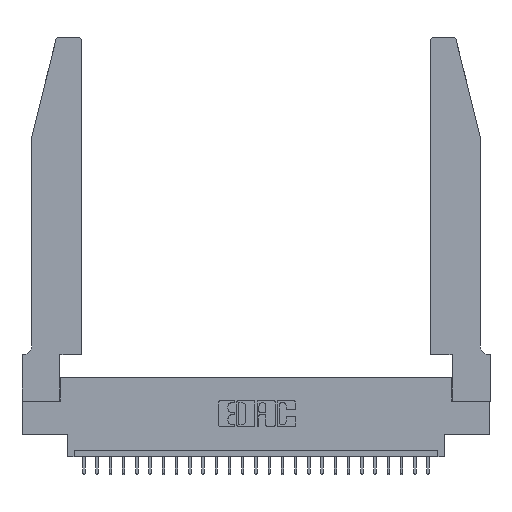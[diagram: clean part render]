
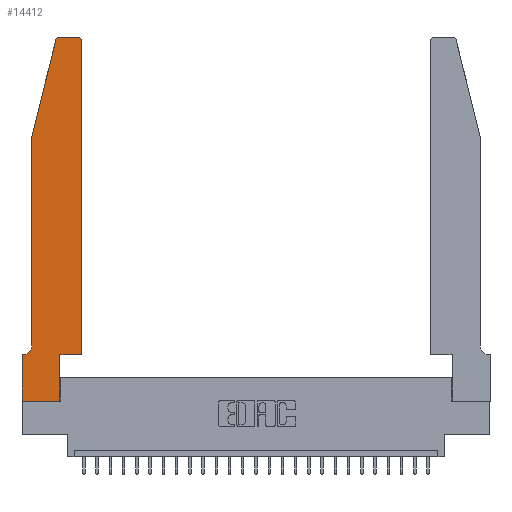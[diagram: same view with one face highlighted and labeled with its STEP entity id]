
A CAD part, top view. The second image highlights one B-rep face of the part: STEP entity #14412.
In plain terms, the highlighted planar face has unit normal (0, 0, 1).
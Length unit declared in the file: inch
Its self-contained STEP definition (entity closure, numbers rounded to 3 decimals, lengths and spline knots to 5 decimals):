
#341 = DIRECTION ( 'NONE',  ( 0., -1., 0. ) ) ;
#376 = ORIENTED_EDGE ( 'NONE', *, *, #8620, .T. ) ;
#528 = AXIS2_PLACEMENT_3D ( 'NONE', #14301, #6112, #1707 ) ;
#694 = EDGE_CURVE ( 'NONE', #7402, #24415, #25344, .T. ) ;
#787 = DIRECTION ( 'NONE',  ( -1., 0., 0. ) ) ;
#813 = CIRCLE ( 'NONE', #26878, 0.03 ) ;
#1213 = ORIENTED_EDGE ( 'NONE', *, *, #19208, .T. ) ;
#1426 = ORIENTED_EDGE ( 'NONE', *, *, #20677, .T. ) ;
#1485 = DIRECTION ( 'NONE',  ( 0., 1., 0. ) ) ;
#1707 = DIRECTION ( 'NONE',  ( 1., 0., 0. ) ) ;
#2209 = VERTEX_POINT ( 'NONE', #5095 ) ;
#2527 = CARTESIAN_POINT ( 'NONE',  ( 0.0755, 2., 0.37 ) ) ;
#3108 = VECTOR ( 'NONE', #8876, 39.37008 ) ;
#3125 = VECTOR ( 'NONE', #4158, 39.37008 ) ;
#3211 = EDGE_CURVE ( 'NONE', #4930, #22419, #3374, .T. ) ;
#3374 = LINE ( 'NONE', #16077, #22943 ) ;
#3645 = CARTESIAN_POINT ( 'NONE',  ( 0.2865, 0.35, 0.37 ) ) ;
#3702 = DIRECTION ( 'NONE',  ( -1., 0., 0. ) ) ;
#3962 = AXIS2_PLACEMENT_3D ( 'NONE', #18215, #22082, #3702 ) ;
#4158 = DIRECTION ( 'NONE',  ( -1., 0., 0. ) ) ;
#4218 = LINE ( 'NONE', #25383, #10726 ) ;
#4930 = VERTEX_POINT ( 'NONE', #3645 ) ;
#5095 = CARTESIAN_POINT ( 'NONE',  ( 0., 0., 0.37 ) ) ;
#5184 = EDGE_LOOP ( 'NONE', ( #8796, #376, #10819, #16436, #1213, #1426, #23191, #9444, #22087, #20140, #8868, #13219 ) ) ;
#5311 = CARTESIAN_POINT ( 'NONE',  ( 0.0755, 0.42, 0.37 ) ) ;
#5367 = LINE ( 'NONE', #26244, #21710 ) ;
#5910 = CARTESIAN_POINT ( 'NONE',  ( 0.4505, 0.35, 0.37 ) ) ;
#5990 = FACE_OUTER_BOUND ( 'NONE', #5184, .T. ) ;
#6112 = DIRECTION ( 'NONE',  ( 0., 0., 1. ) ) ;
#6218 = AXIS2_PLACEMENT_3D ( 'NONE', #20593, #25018, #20462 ) ;
#7402 = VERTEX_POINT ( 'NONE', #24793 ) ;
#7580 = VECTOR ( 'NONE', #14351, 39.37008 ) ;
#7696 = LINE ( 'NONE', #26513, #27016 ) ;
#8125 = VERTEX_POINT ( 'NONE', #22110 ) ;
#8146 = VERTEX_POINT ( 'NONE', #24330 ) ;
#8329 = DIRECTION ( 'NONE',  ( 1., 0., 0. ) ) ;
#8620 = EDGE_CURVE ( 'NONE', #8125, #7402, #813, .T. ) ;
#8796 = ORIENTED_EDGE ( 'NONE', *, *, #23395, .T. ) ;
#8868 = ORIENTED_EDGE ( 'NONE', *, *, #8987, .T. ) ;
#8876 = DIRECTION ( 'NONE',  ( -0.239, -0.971, 0. ) ) ;
#8987 = EDGE_CURVE ( 'NONE', #22419, #26994, #13859, .T. ) ;
#9112 = CARTESIAN_POINT ( 'NONE',  ( 0., 0.35, 0.37 ) ) ;
#9408 = VERTEX_POINT ( 'NONE', #16289 ) ;
#9444 = ORIENTED_EDGE ( 'NONE', *, *, #15350, .T. ) ;
#10726 = VECTOR ( 'NONE', #22778, 39.37008 ) ;
#10819 = ORIENTED_EDGE ( 'NONE', *, *, #694, .T. ) ;
#10979 = VECTOR ( 'NONE', #20210, 39.37008 ) ;
#11382 = VERTEX_POINT ( 'NONE', #5311 ) ;
#11753 = CARTESIAN_POINT ( 'NONE',  ( 0.0755, 2., 0.37 ) ) ;
#12168 = EDGE_CURVE ( 'NONE', #9408, #4930, #7696, .T. ) ;
#13219 = ORIENTED_EDGE ( 'NONE', *, *, #20774, .T. ) ;
#13859 = LINE ( 'NONE', #18417, #10979 ) ;
#14130 = EDGE_CURVE ( 'NONE', #21813, #2209, #21757, .T. ) ;
#14301 = CARTESIAN_POINT ( 'NONE',  ( 0., 0.35, 0.37 ) ) ;
#14351 = DIRECTION ( 'NONE',  ( 0., -1., 0. ) ) ;
#14412 = ADVANCED_FACE ( 'NONE', ( #5990 ), #18855, .T. ) ;
#15219 = LINE ( 'NONE', #19514, #3125 ) ;
#15350 = EDGE_CURVE ( 'NONE', #2209, #9408, #4218, .T. ) ;
#16077 = CARTESIAN_POINT ( 'NONE',  ( 0.4505, 0.35, 0.37 ) ) ;
#16289 = CARTESIAN_POINT ( 'NONE',  ( 0.2865, 0., 0.37 ) ) ;
#16350 = CARTESIAN_POINT ( 'NONE',  ( 0.4505, 2.72, 0.37 ) ) ;
#16436 = ORIENTED_EDGE ( 'NONE', *, *, #23524, .T. ) ;
#18215 = CARTESIAN_POINT ( 'NONE',  ( 0.0055, 0.42, 0.37 ) ) ;
#18417 = CARTESIAN_POINT ( 'NONE',  ( 0.4505, 0.35, 0.37 ) ) ;
#18497 = CARTESIAN_POINT ( 'NONE',  ( 0.0755, 2., 0.37 ) ) ;
#18855 = PLANE ( 'NONE',  #528 ) ;
#19208 = EDGE_CURVE ( 'NONE', #11382, #22347, #20739, .T. ) ;
#19514 = CARTESIAN_POINT ( 'NONE',  ( 0.0755, 0.35, 0.37 ) ) ;
#20100 = DIRECTION ( 'NONE',  ( 1., 0., 0. ) ) ;
#20140 = ORIENTED_EDGE ( 'NONE', *, *, #3211, .T. ) ;
#20210 = DIRECTION ( 'NONE',  ( 0., 1., 0. ) ) ;
#20462 = DIRECTION ( 'NONE',  ( 1., 0., 0. ) ) ;
#20593 = CARTESIAN_POINT ( 'NONE',  ( 0.4205, 2.72, 0.37 ) ) ;
#20677 = EDGE_CURVE ( 'NONE', #22347, #21813, #15219, .T. ) ;
#20739 = CIRCLE ( 'NONE', #3962, 0.07 ) ;
#20774 = EDGE_CURVE ( 'NONE', #26994, #8146, #22119, .T. ) ;
#20840 = VECTOR ( 'NONE', #341, 39.37008 ) ;
#20933 = CARTESIAN_POINT ( 'NONE',  ( 0.284, 2.72, 0.37 ) ) ;
#21356 = CARTESIAN_POINT ( 'NONE',  ( 0., 0., 0.37 ) ) ;
#21710 = VECTOR ( 'NONE', #787, 39.37008 ) ;
#21757 = LINE ( 'NONE', #21356, #20840 ) ;
#21813 = VERTEX_POINT ( 'NONE', #9112 ) ;
#22082 = DIRECTION ( 'NONE',  ( 0., 0., -1. ) ) ;
#22087 = ORIENTED_EDGE ( 'NONE', *, *, #12168, .T. ) ;
#22110 = CARTESIAN_POINT ( 'NONE',  ( 0.284, 2.75, 0.37 ) ) ;
#22119 = CIRCLE ( 'NONE', #6218, 0.03 ) ;
#22347 = VERTEX_POINT ( 'NONE', #24709 ) ;
#22419 = VERTEX_POINT ( 'NONE', #5910 ) ;
#22778 = DIRECTION ( 'NONE',  ( 1., 0., 0. ) ) ;
#22943 = VECTOR ( 'NONE', #20100, 39.37008 ) ;
#23191 = ORIENTED_EDGE ( 'NONE', *, *, #14130, .T. ) ;
#23395 = EDGE_CURVE ( 'NONE', #8146, #8125, #5367, .T. ) ;
#23524 = EDGE_CURVE ( 'NONE', #24415, #11382, #24856, .T. ) ;
#24330 = CARTESIAN_POINT ( 'NONE',  ( 0.4205, 2.75, 0.37 ) ) ;
#24415 = VERTEX_POINT ( 'NONE', #11753 ) ;
#24709 = CARTESIAN_POINT ( 'NONE',  ( 0.0055, 0.35, 0.37 ) ) ;
#24793 = CARTESIAN_POINT ( 'NONE',  ( 0.25487, 2.72718, 0.37 ) ) ;
#24856 = LINE ( 'NONE', #18497, #7580 ) ;
#25018 = DIRECTION ( 'NONE',  ( 0., 0., 1. ) ) ;
#25344 = LINE ( 'NONE', #2527, #3108 ) ;
#25383 = CARTESIAN_POINT ( 'NONE',  ( 0., 0., 0.37 ) ) ;
#26244 = CARTESIAN_POINT ( 'NONE',  ( 0.2605, 2.75, 0.37 ) ) ;
#26513 = CARTESIAN_POINT ( 'NONE',  ( 0.2865, 0.35, 0.37 ) ) ;
#26878 = AXIS2_PLACEMENT_3D ( 'NONE', #20933, #27282, #8329 ) ;
#26994 = VERTEX_POINT ( 'NONE', #16350 ) ;
#27016 = VECTOR ( 'NONE', #1485, 39.37008 ) ;
#27282 = DIRECTION ( 'NONE',  ( 0., 0., 1. ) ) ;
